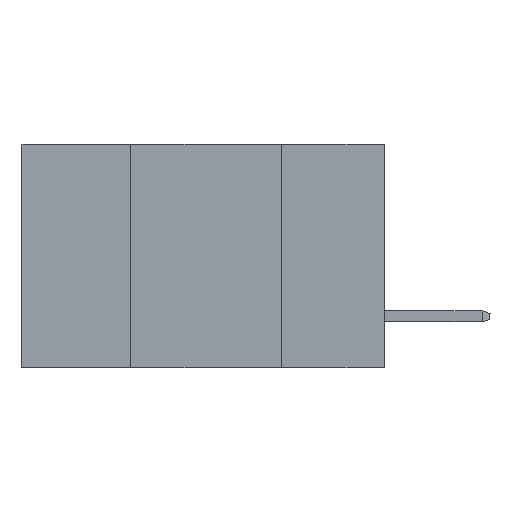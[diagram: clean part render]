
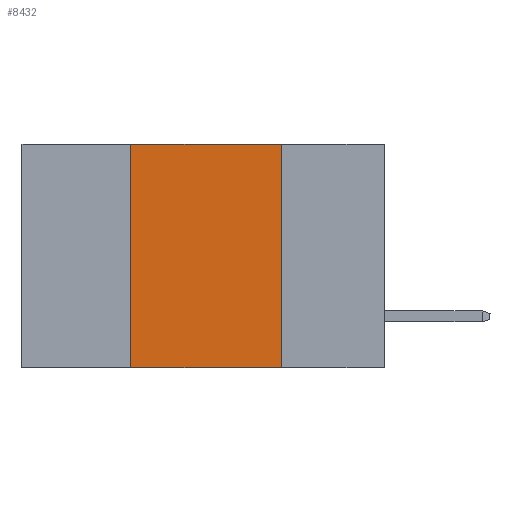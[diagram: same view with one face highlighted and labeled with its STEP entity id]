
A CAD part, left-side view. The second image highlights one B-rep face of the part: STEP entity #8432.
In plain terms, the highlighted planar face has unit normal (-1, 0, 0).
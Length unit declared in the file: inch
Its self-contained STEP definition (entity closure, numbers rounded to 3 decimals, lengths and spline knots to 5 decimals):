
#320 = LINE ( 'NONE', #521, #635 ) ;
#521 = CARTESIAN_POINT ( 'NONE',  ( 0., 0.6, -0.37 ) ) ;
#635 = VECTOR ( 'NONE', #4498, 39.37008 ) ;
#751 = LINE ( 'NONE', #3779, #2070 ) ;
#1438 = EDGE_CURVE ( 'NONE', #5308, #7528, #8898, .T. ) ;
#1477 = EDGE_CURVE ( 'NONE', #5308, #10020, #320, .T. ) ;
#1677 = EDGE_CURVE ( 'NONE', #8777, #10020, #5634, .T. ) ;
#1700 = CARTESIAN_POINT ( 'NONE',  ( 0., 0.17, -0.37 ) ) ;
#1818 = CARTESIAN_POINT ( 'NONE',  ( 0., 0.42, -0.37 ) ) ;
#2070 = VECTOR ( 'NONE', #8495, 39.37008 ) ;
#2626 = FACE_OUTER_BOUND ( 'NONE', #6913, .T. ) ;
#2674 = DIRECTION ( 'NONE',  ( 0., 0., -1. ) ) ;
#3455 = DIRECTION ( 'NONE',  ( 1., 0., 0. ) ) ;
#3495 = CARTESIAN_POINT ( 'NONE',  ( 0., 0.17, -0.37 ) ) ;
#3779 = CARTESIAN_POINT ( 'NONE',  ( 0., 0.6, 0. ) ) ;
#4246 = DIRECTION ( 'NONE',  ( 0., 0., 1. ) ) ;
#4498 = DIRECTION ( 'NONE',  ( 0., -1., 0. ) ) ;
#4927 = VECTOR ( 'NONE', #4246, 39.37008 ) ;
#5042 = VECTOR ( 'NONE', #9611, 39.37008 ) ;
#5308 = VERTEX_POINT ( 'NONE', #5421 ) ;
#5421 = CARTESIAN_POINT ( 'NONE',  ( 0., 0.42, -0.37 ) ) ;
#5634 = LINE ( 'NONE', #1700, #5042 ) ;
#5777 = PLANE ( 'NONE',  #7487 ) ;
#6369 = ORIENTED_EDGE ( 'NONE', *, *, #1438, .F. ) ;
#6594 = CARTESIAN_POINT ( 'NONE',  ( 0., 0.6, 0. ) ) ;
#6913 = EDGE_LOOP ( 'NONE', ( #8293, #9844, #6369, #6937 ) ) ;
#6937 = ORIENTED_EDGE ( 'NONE', *, *, #1477, .T. ) ;
#7436 = CARTESIAN_POINT ( 'NONE',  ( 0., 0.17, 0. ) ) ;
#7487 = AXIS2_PLACEMENT_3D ( 'NONE', #6594, #3455, #2674 ) ;
#7528 = VERTEX_POINT ( 'NONE', #8907 ) ;
#8027 = EDGE_CURVE ( 'NONE', #7528, #8777, #751, .T. ) ;
#8293 = ORIENTED_EDGE ( 'NONE', *, *, #1677, .F. ) ;
#8432 = ADVANCED_FACE ( 'NONE', ( #2626 ), #5777, .F. ) ;
#8495 = DIRECTION ( 'NONE',  ( 0., -1., 0. ) ) ;
#8777 = VERTEX_POINT ( 'NONE', #7436 ) ;
#8898 = LINE ( 'NONE', #1818, #4927 ) ;
#8907 = CARTESIAN_POINT ( 'NONE',  ( 0., 0.42, 0. ) ) ;
#9611 = DIRECTION ( 'NONE',  ( 0., 0., -1. ) ) ;
#9844 = ORIENTED_EDGE ( 'NONE', *, *, #8027, .F. ) ;
#10020 = VERTEX_POINT ( 'NONE', #3495 ) ;
